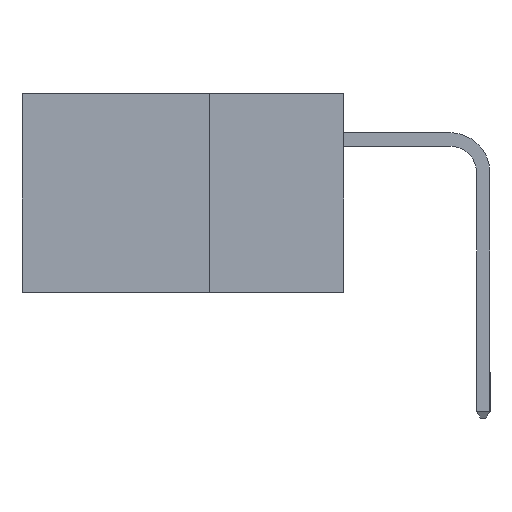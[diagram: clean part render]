
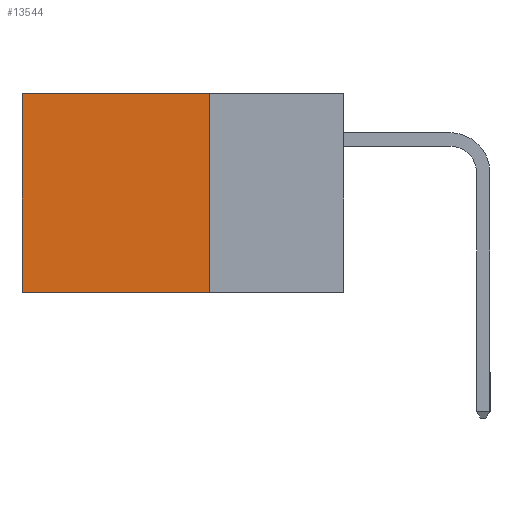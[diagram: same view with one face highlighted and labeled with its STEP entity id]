
A CAD part, left-side view. The second image highlights one B-rep face of the part: STEP entity #13544.
In plain terms, the highlighted planar face has unit normal (-1, 0, 0).
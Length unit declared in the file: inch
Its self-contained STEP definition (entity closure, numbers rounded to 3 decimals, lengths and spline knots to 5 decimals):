
#2931 = EDGE_CURVE ( 'NONE', #15118, #5875, #20345, .T. ) ;
#4069 = EDGE_CURVE ( 'NONE', #18232, #5875, #12722, .T. ) ;
#4107 = VECTOR ( 'NONE', #17889, 39.37008 ) ;
#4589 = DIRECTION ( 'NONE',  ( 0., 1., 0. ) ) ;
#4896 = LINE ( 'NONE', #5944, #8433 ) ;
#5064 = CARTESIAN_POINT ( 'NONE',  ( 0.298, 0.6, 0. ) ) ;
#5443 = CARTESIAN_POINT ( 'NONE',  ( 0.298, 0.6, 0. ) ) ;
#5538 = EDGE_LOOP ( 'NONE', ( #16387, #8967, #10832, #13740 ) ) ;
#5875 = VERTEX_POINT ( 'NONE', #17321 ) ;
#5944 = CARTESIAN_POINT ( 'NONE',  ( 0.298, 0.25, 0. ) ) ;
#7422 = DIRECTION ( 'NONE',  ( 0., 0., -1. ) ) ;
#7563 = DIRECTION ( 'NONE',  ( 0., 1., 0. ) ) ;
#8433 = VECTOR ( 'NONE', #7563, 39.37008 ) ;
#8967 = ORIENTED_EDGE ( 'NONE', *, *, #2931, .F. ) ;
#10832 = ORIENTED_EDGE ( 'NONE', *, *, #20216, .F. ) ;
#12442 = DIRECTION ( 'NONE',  ( 1., 0., 0. ) ) ;
#12663 = CARTESIAN_POINT ( 'NONE',  ( 0.298, 0.25, -0.37 ) ) ;
#12708 = AXIS2_PLACEMENT_3D ( 'NONE', #17377, #12442, #13964 ) ;
#12722 = LINE ( 'NONE', #5064, #4107 ) ;
#13037 = EDGE_CURVE ( 'NONE', #13611, #18232, #4896, .T. ) ;
#13544 = ADVANCED_FACE ( 'NONE', ( #16466 ), #17448, .F. ) ;
#13611 = VERTEX_POINT ( 'NONE', #16013 ) ;
#13740 = ORIENTED_EDGE ( 'NONE', *, *, #13037, .T. ) ;
#13778 = VECTOR ( 'NONE', #4589, 39.37008 ) ;
#13964 = DIRECTION ( 'NONE',  ( 0., 0., -1. ) ) ;
#15118 = VERTEX_POINT ( 'NONE', #12663 ) ;
#16013 = CARTESIAN_POINT ( 'NONE',  ( 0.298, 0.25, 0. ) ) ;
#16232 = LINE ( 'NONE', #18632, #16730 ) ;
#16387 = ORIENTED_EDGE ( 'NONE', *, *, #4069, .T. ) ;
#16466 = FACE_OUTER_BOUND ( 'NONE', #5538, .T. ) ;
#16730 = VECTOR ( 'NONE', #7422, 39.37008 ) ;
#17321 = CARTESIAN_POINT ( 'NONE',  ( 0.298, 0.6, -0.37 ) ) ;
#17377 = CARTESIAN_POINT ( 'NONE',  ( 0.298, 0.25, 0. ) ) ;
#17448 = PLANE ( 'NONE',  #12708 ) ;
#17889 = DIRECTION ( 'NONE',  ( 0., 0., -1. ) ) ;
#18232 = VERTEX_POINT ( 'NONE', #5443 ) ;
#18632 = CARTESIAN_POINT ( 'NONE',  ( 0.298, 0.25, 0. ) ) ;
#20216 = EDGE_CURVE ( 'NONE', #13611, #15118, #16232, .T. ) ;
#20345 = LINE ( 'NONE', #20726, #13778 ) ;
#20726 = CARTESIAN_POINT ( 'NONE',  ( 0.298, 0.25, -0.37 ) ) ;
